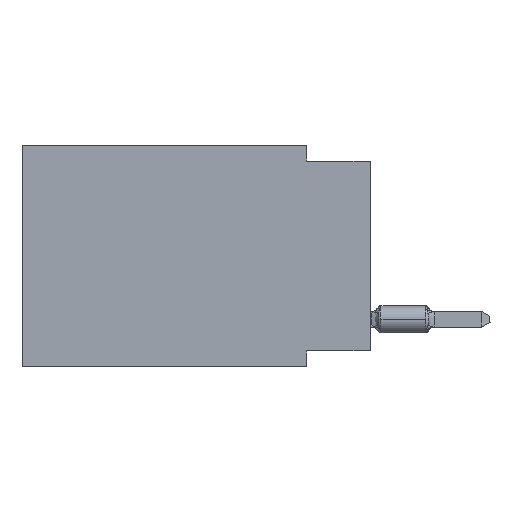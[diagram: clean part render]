
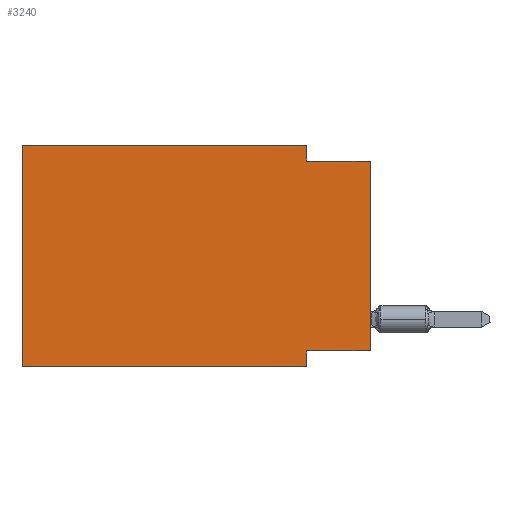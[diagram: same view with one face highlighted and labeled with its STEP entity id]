
A CAD part, left-side view. The second image highlights one B-rep face of the part: STEP entity #3240.
In plain terms, the highlighted planar face has unit normal (-1, 0, 0).
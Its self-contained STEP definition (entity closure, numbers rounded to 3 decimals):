
#18 = CARTESIAN_POINT ( 'NONE',  ( 0., 0., 0. ) ) ;
#25 = CARTESIAN_POINT ( 'NONE',  ( 0., 2.54, -8.255 ) ) ;
#46 = ORIENTED_EDGE ( 'NONE', *, *, #916, .T. ) ;
#511 = CARTESIAN_POINT ( 'NONE',  ( 0., 2.54, -0.635 ) ) ;
#767 = CARTESIAN_POINT ( 'NONE',  ( 0., 2.54, -8.89 ) ) ;
#916 = EDGE_CURVE ( 'NONE', #3046, #14656, #1616, .T. ) ;
#1414 = VECTOR ( 'NONE', #12333, 1000. ) ;
#1616 = LINE ( 'NONE', #18, #9381 ) ;
#1618 = VERTEX_POINT ( 'NONE', #15315 ) ;
#1625 = CARTESIAN_POINT ( 'NONE',  ( 0., 13.97, 0. ) ) ;
#1744 = VECTOR ( 'NONE', #7796, 1000. ) ;
#2193 = LINE ( 'NONE', #8723, #8597 ) ;
#2425 = ORIENTED_EDGE ( 'NONE', *, *, #9801, .F. ) ;
#2775 = CARTESIAN_POINT ( 'NONE',  ( 0., 0., -8.255 ) ) ;
#3010 = VECTOR ( 'NONE', #7614, 1000. ) ;
#3046 = VERTEX_POINT ( 'NONE', #17348 ) ;
#3169 = VECTOR ( 'NONE', #7338, 1000. ) ;
#3240 = ADVANCED_FACE ( 'NONE', ( #5113 ), #11636, .F. ) ;
#3511 = VECTOR ( 'NONE', #11981, 1000. ) ;
#4014 = VERTEX_POINT ( 'NONE', #1625 ) ;
#5112 = ORIENTED_EDGE ( 'NONE', *, *, #5362, .F. ) ;
#5113 = FACE_OUTER_BOUND ( 'NONE', #18373, .T. ) ;
#5285 = CARTESIAN_POINT ( 'NONE',  ( 0., 13.97, 0. ) ) ;
#5362 = EDGE_CURVE ( 'NONE', #3046, #9625, #9197, .T. ) ;
#5443 = LINE ( 'NONE', #5554, #3511 ) ;
#5554 = CARTESIAN_POINT ( 'NONE',  ( 0., 2.54, 0. ) ) ;
#6809 = VERTEX_POINT ( 'NONE', #14938 ) ;
#7027 = VERTEX_POINT ( 'NONE', #15167 ) ;
#7301 = LINE ( 'NONE', #19181, #3010 ) ;
#7338 = DIRECTION ( 'NONE',  ( 0., -1., 0. ) ) ;
#7428 = AXIS2_PLACEMENT_3D ( 'NONE', #15944, #17660, #20977 ) ;
#7614 = DIRECTION ( 'NONE',  ( 0., -1., 0. ) ) ;
#7796 = DIRECTION ( 'NONE',  ( 0., 1., 0. ) ) ;
#8597 = VECTOR ( 'NONE', #20595, 1000. ) ;
#8723 = CARTESIAN_POINT ( 'NONE',  ( 0., 0., -0.635 ) ) ;
#8807 = LINE ( 'NONE', #767, #1414 ) ;
#9197 = LINE ( 'NONE', #2775, #1744 ) ;
#9381 = VECTOR ( 'NONE', #9965, 1000. ) ;
#9625 = VERTEX_POINT ( 'NONE', #25 ) ;
#9801 = EDGE_CURVE ( 'NONE', #4014, #7027, #7301, .T. ) ;
#9965 = DIRECTION ( 'NONE',  ( 0., 0., 1. ) ) ;
#10930 = ORIENTED_EDGE ( 'NONE', *, *, #14178, .F. ) ;
#11636 = PLANE ( 'NONE',  #7428 ) ;
#11956 = CARTESIAN_POINT ( 'NONE',  ( 0., 13.97, -8.89 ) ) ;
#11981 = DIRECTION ( 'NONE',  ( 0., 0., -1. ) ) ;
#12333 = DIRECTION ( 'NONE',  ( 0., 0., -1. ) ) ;
#12348 = VERTEX_POINT ( 'NONE', #511 ) ;
#12581 = ORIENTED_EDGE ( 'NONE', *, *, #17600, .F. ) ;
#13765 = ORIENTED_EDGE ( 'NONE', *, *, #14936, .F. ) ;
#14178 = EDGE_CURVE ( 'NONE', #7027, #12348, #5443, .T. ) ;
#14648 = ORIENTED_EDGE ( 'NONE', *, *, #17104, .F. ) ;
#14656 = VERTEX_POINT ( 'NONE', #17074 ) ;
#14739 = EDGE_CURVE ( 'NONE', #1618, #6809, #20080, .T. ) ;
#14801 = DIRECTION ( 'NONE',  ( 0., 0., 1. ) ) ;
#14936 = EDGE_CURVE ( 'NONE', #1618, #4014, #19624, .T. ) ;
#14938 = CARTESIAN_POINT ( 'NONE',  ( 0., 2.54, -8.89 ) ) ;
#15167 = CARTESIAN_POINT ( 'NONE',  ( 0., 2.54, 0. ) ) ;
#15315 = CARTESIAN_POINT ( 'NONE',  ( 0., 13.97, -8.89 ) ) ;
#15515 = ORIENTED_EDGE ( 'NONE', *, *, #14739, .T. ) ;
#15944 = CARTESIAN_POINT ( 'NONE',  ( 0., 13.97, 0. ) ) ;
#17074 = CARTESIAN_POINT ( 'NONE',  ( 0., 0., -0.635 ) ) ;
#17104 = EDGE_CURVE ( 'NONE', #12348, #14656, #2193, .T. ) ;
#17348 = CARTESIAN_POINT ( 'NONE',  ( 0., 0., -8.255 ) ) ;
#17600 = EDGE_CURVE ( 'NONE', #9625, #6809, #8807, .T. ) ;
#17660 = DIRECTION ( 'NONE',  ( 1., 0., 0. ) ) ;
#18255 = VECTOR ( 'NONE', #14801, 1000. ) ;
#18373 = EDGE_LOOP ( 'NONE', ( #46, #14648, #10930, #2425, #13765, #15515, #12581, #5112 ) ) ;
#19181 = CARTESIAN_POINT ( 'NONE',  ( 0., 13.97, 0. ) ) ;
#19624 = LINE ( 'NONE', #5285, #18255 ) ;
#20080 = LINE ( 'NONE', #11956, #3169 ) ;
#20595 = DIRECTION ( 'NONE',  ( 0., -1., 0. ) ) ;
#20977 = DIRECTION ( 'NONE',  ( 0., 0., -1. ) ) ;
